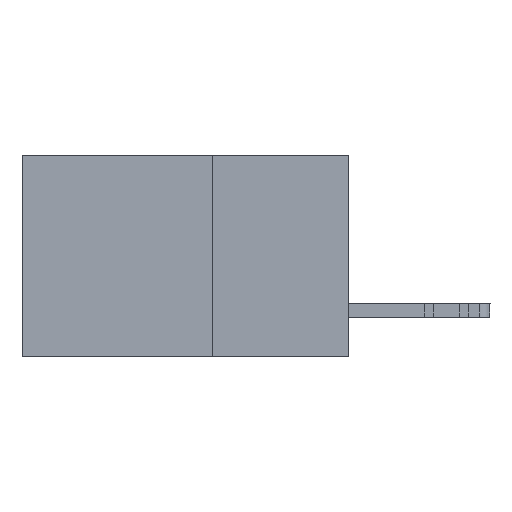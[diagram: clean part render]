
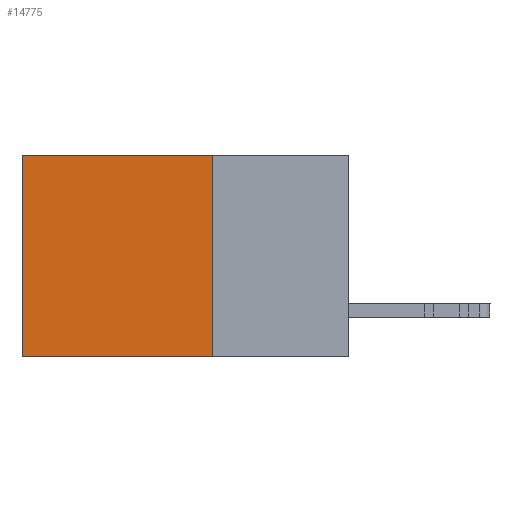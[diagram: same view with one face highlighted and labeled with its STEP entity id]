
A CAD part, left-side view. The second image highlights one B-rep face of the part: STEP entity #14775.
In plain terms, the highlighted planar face has unit normal (-1, 0, 0).
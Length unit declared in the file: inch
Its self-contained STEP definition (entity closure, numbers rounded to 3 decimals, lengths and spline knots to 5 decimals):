
#420 = CARTESIAN_POINT ( 'NONE',  ( 0.2615, 0.25, -0.37 ) ) ;
#749 = DIRECTION ( 'NONE',  ( 0., 0., -1. ) ) ;
#2428 = LINE ( 'NONE', #22833, #22074 ) ;
#2502 = VECTOR ( 'NONE', #21675, 39.37008 ) ;
#2626 = CARTESIAN_POINT ( 'NONE',  ( 0.2615, 0.25, -0.37 ) ) ;
#2685 = VERTEX_POINT ( 'NONE', #19497 ) ;
#3062 = DIRECTION ( 'NONE',  ( 0., 0., -1. ) ) ;
#4435 = EDGE_CURVE ( 'NONE', #12556, #2685, #2428, .T. ) ;
#4612 = CARTESIAN_POINT ( 'NONE',  ( 0.2615, 0.25, -0.37 ) ) ;
#4645 = CARTESIAN_POINT ( 'NONE',  ( 0.2615, 0.25, -0.37 ) ) ;
#7400 = VECTOR ( 'NONE', #3062, 39.37008 ) ;
#8651 = LINE ( 'NONE', #2626, #23565 ) ;
#9369 = FACE_OUTER_BOUND ( 'NONE', #14402, .T. ) ;
#10166 = EDGE_CURVE ( 'NONE', #12556, #17346, #8651, .T. ) ;
#10588 = PLANE ( 'NONE',  #19572 ) ;
#10649 = VERTEX_POINT ( 'NONE', #23649 ) ;
#12450 = DIRECTION ( 'NONE',  ( 1., 0., 0. ) ) ;
#12556 = VERTEX_POINT ( 'NONE', #22116 ) ;
#14230 = ORIENTED_EDGE ( 'NONE', *, *, #10166, .F. ) ;
#14402 = EDGE_LOOP ( 'NONE', ( #21642, #22201, #14230, #14864 ) ) ;
#14775 = ADVANCED_FACE ( 'NONE', ( #9369 ), #10588, .F. ) ;
#14864 = ORIENTED_EDGE ( 'NONE', *, *, #4435, .T. ) ;
#16178 = DIRECTION ( 'NONE',  ( 0., 0., -1. ) ) ;
#16580 = CARTESIAN_POINT ( 'NONE',  ( 0.2615, 0.6, -0.37 ) ) ;
#17346 = VERTEX_POINT ( 'NONE', #420 ) ;
#17895 = LINE ( 'NONE', #4612, #2502 ) ;
#18086 = EDGE_CURVE ( 'NONE', #2685, #10649, #21794, .T. ) ;
#19497 = CARTESIAN_POINT ( 'NONE',  ( 0.2615, 0.6, 0. ) ) ;
#19572 = AXIS2_PLACEMENT_3D ( 'NONE', #4645, #12450, #749 ) ;
#21642 = ORIENTED_EDGE ( 'NONE', *, *, #18086, .T. ) ;
#21675 = DIRECTION ( 'NONE',  ( 0., 1., 0. ) ) ;
#21794 = LINE ( 'NONE', #16580, #7400 ) ;
#22074 = VECTOR ( 'NONE', #22781, 39.37008 ) ;
#22110 = EDGE_CURVE ( 'NONE', #17346, #10649, #17895, .T. ) ;
#22116 = CARTESIAN_POINT ( 'NONE',  ( 0.2615, 0.25, 0. ) ) ;
#22201 = ORIENTED_EDGE ( 'NONE', *, *, #22110, .F. ) ;
#22781 = DIRECTION ( 'NONE',  ( 0., 1., 0. ) ) ;
#22833 = CARTESIAN_POINT ( 'NONE',  ( 0.2615, 0.25, 0. ) ) ;
#23565 = VECTOR ( 'NONE', #16178, 39.37008 ) ;
#23649 = CARTESIAN_POINT ( 'NONE',  ( 0.2615, 0.6, -0.37 ) ) ;
